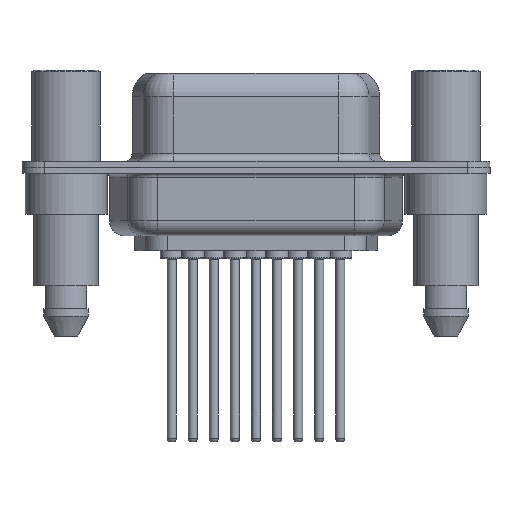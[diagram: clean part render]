
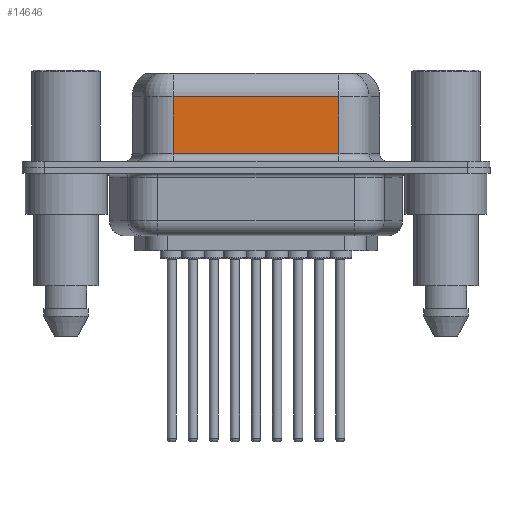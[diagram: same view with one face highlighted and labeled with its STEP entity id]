
A CAD part, front view. The second image highlights one B-rep face of the part: STEP entity #14646.
In plain terms, the highlighted planar face has unit normal (0, -1, 0).
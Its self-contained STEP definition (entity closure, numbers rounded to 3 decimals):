
#263 = VERTEX_POINT ( 'NONE', #13315 ) ;
#498 = EDGE_LOOP ( 'NONE', ( #15248, #6842, #5680, #10642 ) ) ;
#2136 = VERTEX_POINT ( 'NONE', #15080 ) ;
#2300 = CARTESIAN_POINT ( 'NONE',  ( 7.038, -3.95, 4.65 ) ) ;
#2311 = DIRECTION ( 'NONE',  ( 0., 0., -1. ) ) ;
#2701 = VECTOR ( 'NONE', #6753, 1000. ) ;
#2794 = EDGE_CURVE ( 'NONE', #13051, #2136, #8235, .T. ) ;
#3058 = LINE ( 'NONE', #14038, #2701 ) ;
#3659 = LINE ( 'NONE', #13295, #4017 ) ;
#3788 = EDGE_CURVE ( 'NONE', #263, #13051, #10605, .T. ) ;
#4017 = VECTOR ( 'NONE', #2311, 1000. ) ;
#4428 = EDGE_CURVE ( 'NONE', #263, #13929, #3659, .T. ) ;
#4824 = VECTOR ( 'NONE', #6891, 1000. ) ;
#5017 = AXIS2_PLACEMENT_3D ( 'NONE', #13132, #7944, #11606 ) ;
#5680 = ORIENTED_EDGE ( 'NONE', *, *, #2794, .T. ) ;
#6739 = FACE_OUTER_BOUND ( 'NONE', #498, .T. ) ;
#6753 = DIRECTION ( 'NONE',  ( 1., 0., 0. ) ) ;
#6842 = ORIENTED_EDGE ( 'NONE', *, *, #3788, .T. ) ;
#6891 = DIRECTION ( 'NONE',  ( 0., 0., -1. ) ) ;
#7814 = CARTESIAN_POINT ( 'NONE',  ( 17.962, -3.95, 0.9 ) ) ;
#7944 = DIRECTION ( 'NONE',  ( 0., 1., 0. ) ) ;
#8235 = LINE ( 'NONE', #14329, #4824 ) ;
#8248 = PLANE ( 'NONE',  #5017 ) ;
#9546 = DIRECTION ( 'NONE',  ( -1., 0., 0. ) ) ;
#10605 = LINE ( 'NONE', #13019, #14781 ) ;
#10634 = EDGE_CURVE ( 'NONE', #2136, #13929, #3058, .T. ) ;
#10642 = ORIENTED_EDGE ( 'NONE', *, *, #10634, .T. ) ;
#11606 = DIRECTION ( 'NONE',  ( 0., 0., 1. ) ) ;
#13019 = CARTESIAN_POINT ( 'NONE',  ( 17.962, -3.95, 4.65 ) ) ;
#13051 = VERTEX_POINT ( 'NONE', #2300 ) ;
#13132 = CARTESIAN_POINT ( 'NONE',  ( 17.962, -3.95, 6.4 ) ) ;
#13295 = CARTESIAN_POINT ( 'NONE',  ( 17.962, -3.95, 6.4 ) ) ;
#13315 = CARTESIAN_POINT ( 'NONE',  ( 17.962, -3.95, 4.65 ) ) ;
#13929 = VERTEX_POINT ( 'NONE', #7814 ) ;
#14038 = CARTESIAN_POINT ( 'NONE',  ( 17.962, -3.95, 0.9 ) ) ;
#14329 = CARTESIAN_POINT ( 'NONE',  ( 7.038, -3.95, 6.4 ) ) ;
#14646 = ADVANCED_FACE ( 'NONE', ( #6739 ), #8248, .F. ) ;
#14781 = VECTOR ( 'NONE', #9546, 1000. ) ;
#15080 = CARTESIAN_POINT ( 'NONE',  ( 7.038, -3.95, 0.9 ) ) ;
#15248 = ORIENTED_EDGE ( 'NONE', *, *, #4428, .F. ) ;
